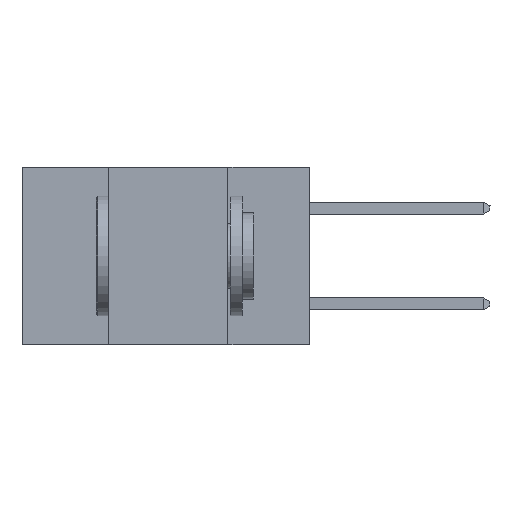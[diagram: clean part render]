
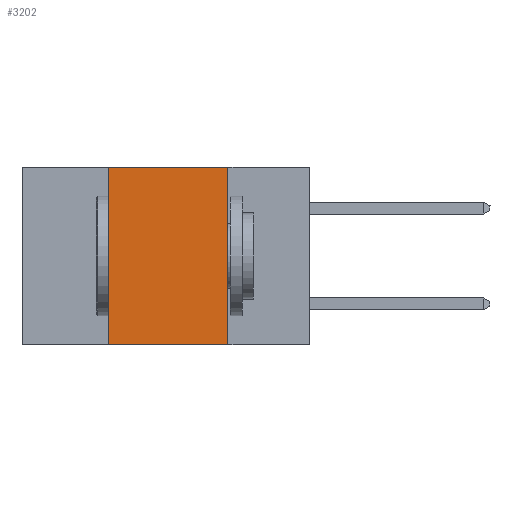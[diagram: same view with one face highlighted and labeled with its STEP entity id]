
A CAD part, left-side view. The second image highlights one B-rep face of the part: STEP entity #3202.
In plain terms, the highlighted planar face has unit normal (-1, 0, 0).
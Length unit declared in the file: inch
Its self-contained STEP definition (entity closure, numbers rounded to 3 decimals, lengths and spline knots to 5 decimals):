
#271 = CARTESIAN_POINT ( 'NONE',  ( 0., 0.42, 0. ) ) ;
#286 = VERTEX_POINT ( 'NONE', #1183 ) ;
#629 = ORIENTED_EDGE ( 'NONE', *, *, #3504, .F. ) ;
#707 = VERTEX_POINT ( 'NONE', #3903 ) ;
#1183 = CARTESIAN_POINT ( 'NONE',  ( 0., 0.42, -0.37 ) ) ;
#2107 = DIRECTION ( 'NONE',  ( 0., -1., 0. ) ) ;
#2317 = VECTOR ( 'NONE', #9787, 39.37008 ) ;
#2645 = VECTOR ( 'NONE', #5371, 39.37008 ) ;
#2905 = EDGE_CURVE ( 'NONE', #286, #707, #10344, .T. ) ;
#3202 = ADVANCED_FACE ( 'NONE', ( #5730 ), #8014, .F. ) ;
#3294 = ORIENTED_EDGE ( 'NONE', *, *, #2905, .T. ) ;
#3345 = ORIENTED_EDGE ( 'NONE', *, *, #8442, .F. ) ;
#3504 = EDGE_CURVE ( 'NONE', #11125, #8897, #10047, .T. ) ;
#3903 = CARTESIAN_POINT ( 'NONE',  ( 0., 0.17, -0.37 ) ) ;
#5371 = DIRECTION ( 'NONE',  ( 0., 0., 1. ) ) ;
#5730 = FACE_OUTER_BOUND ( 'NONE', #6169, .T. ) ;
#6169 = EDGE_LOOP ( 'NONE', ( #3345, #629, #8860, #3294 ) ) ;
#6257 = CARTESIAN_POINT ( 'NONE',  ( 0., 0.42, 0. ) ) ;
#6930 = CARTESIAN_POINT ( 'NONE',  ( 0., 0.6, 0. ) ) ;
#7553 = CARTESIAN_POINT ( 'NONE',  ( 0., 0.17, 0. ) ) ;
#7732 = AXIS2_PLACEMENT_3D ( 'NONE', #8056, #9165, #9121 ) ;
#8014 = PLANE ( 'NONE',  #7732 ) ;
#8056 = CARTESIAN_POINT ( 'NONE',  ( 0., 0.6, 0. ) ) ;
#8401 = VECTOR ( 'NONE', #2107, 39.37008 ) ;
#8442 = EDGE_CURVE ( 'NONE', #8897, #707, #10251, .T. ) ;
#8635 = CARTESIAN_POINT ( 'NONE',  ( 0., 0.6, -0.37 ) ) ;
#8860 = ORIENTED_EDGE ( 'NONE', *, *, #10072, .F. ) ;
#8897 = VERTEX_POINT ( 'NONE', #9643 ) ;
#9121 = DIRECTION ( 'NONE',  ( 0., 0., -1. ) ) ;
#9165 = DIRECTION ( 'NONE',  ( 1., 0., 0. ) ) ;
#9643 = CARTESIAN_POINT ( 'NONE',  ( 0., 0.17, 0. ) ) ;
#9787 = DIRECTION ( 'NONE',  ( 0., -1., 0. ) ) ;
#9967 = VECTOR ( 'NONE', #12299, 39.37008 ) ;
#10047 = LINE ( 'NONE', #6930, #2317 ) ;
#10072 = EDGE_CURVE ( 'NONE', #286, #11125, #10300, .T. ) ;
#10251 = LINE ( 'NONE', #7553, #9967 ) ;
#10300 = LINE ( 'NONE', #6257, #2645 ) ;
#10344 = LINE ( 'NONE', #8635, #8401 ) ;
#11125 = VERTEX_POINT ( 'NONE', #271 ) ;
#12299 = DIRECTION ( 'NONE',  ( 0., 0., -1. ) ) ;
